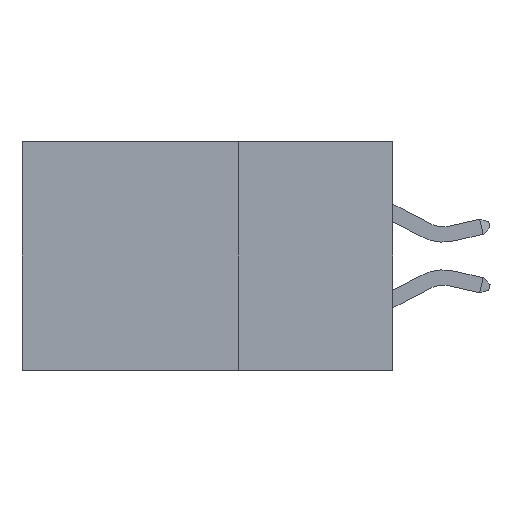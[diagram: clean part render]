
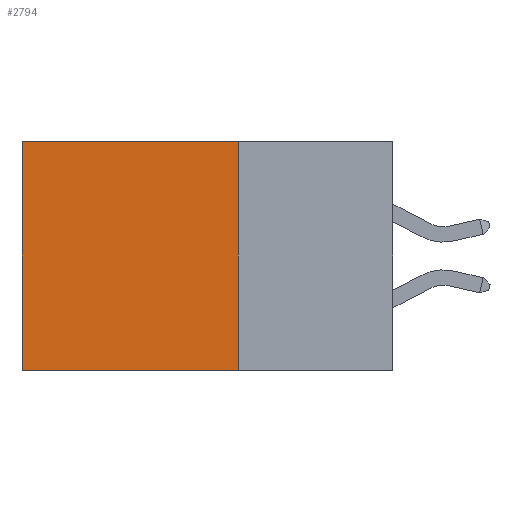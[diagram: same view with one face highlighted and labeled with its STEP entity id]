
A CAD part, left-side view. The second image highlights one B-rep face of the part: STEP entity #2794.
In plain terms, the highlighted planar face has unit normal (-1, 0, 0).
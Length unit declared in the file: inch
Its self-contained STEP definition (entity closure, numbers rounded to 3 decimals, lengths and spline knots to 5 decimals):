
#591 = CARTESIAN_POINT ( 'NONE',  ( 0.2875, 0.6, 0. ) ) ;
#1231 = ORIENTED_EDGE ( 'NONE', *, *, #15293, .T. ) ;
#2356 = DIRECTION ( 'NONE',  ( 0., 0., -1. ) ) ;
#2794 = ADVANCED_FACE ( 'NONE', ( #4543 ), #17885, .F. ) ;
#3355 = VECTOR ( 'NONE', #13983, 39.37008 ) ;
#4543 = FACE_OUTER_BOUND ( 'NONE', #29077, .T. ) ;
#4816 = CARTESIAN_POINT ( 'NONE',  ( 0.2875, 0.25, 0. ) ) ;
#7185 = CARTESIAN_POINT ( 'NONE',  ( 0.2875, 0.25, -0.37 ) ) ;
#7230 = VERTEX_POINT ( 'NONE', #27757 ) ;
#7694 = CARTESIAN_POINT ( 'NONE',  ( 0.2875, 0.6, -0.37 ) ) ;
#7785 = EDGE_CURVE ( 'NONE', #26499, #25138, #21402, .T. ) ;
#8423 = ORIENTED_EDGE ( 'NONE', *, *, #19482, .F. ) ;
#8565 = VECTOR ( 'NONE', #23103, 39.37008 ) ;
#8801 = CARTESIAN_POINT ( 'NONE',  ( 0.2875, 0.25, 0. ) ) ;
#11201 = AXIS2_PLACEMENT_3D ( 'NONE', #8801, #24836, #2356 ) ;
#11332 = DIRECTION ( 'NONE',  ( 0., 0., -1. ) ) ;
#11420 = DIRECTION ( 'NONE',  ( 0., 0., -1. ) ) ;
#12532 = CARTESIAN_POINT ( 'NONE',  ( 0.2875, 0.25, -0.37 ) ) ;
#13983 = DIRECTION ( 'NONE',  ( 0., 1., 0. ) ) ;
#15293 = EDGE_CURVE ( 'NONE', #24431, #25138, #18351, .T. ) ;
#17885 = PLANE ( 'NONE',  #11201 ) ;
#18351 = LINE ( 'NONE', #27538, #22926 ) ;
#19482 = EDGE_CURVE ( 'NONE', #7230, #26499, #23538, .T. ) ;
#21134 = CARTESIAN_POINT ( 'NONE',  ( 0.2875, 0.25, 0. ) ) ;
#21402 = LINE ( 'NONE', #7185, #3355 ) ;
#22926 = VECTOR ( 'NONE', #11420, 39.37008 ) ;
#23103 = DIRECTION ( 'NONE',  ( 0., 1., 0. ) ) ;
#23538 = LINE ( 'NONE', #4816, #24603 ) ;
#23799 = LINE ( 'NONE', #21134, #8565 ) ;
#24389 = EDGE_CURVE ( 'NONE', #7230, #24431, #23799, .T. ) ;
#24431 = VERTEX_POINT ( 'NONE', #591 ) ;
#24603 = VECTOR ( 'NONE', #11332, 39.37008 ) ;
#24836 = DIRECTION ( 'NONE',  ( 1., 0., 0. ) ) ;
#25138 = VERTEX_POINT ( 'NONE', #7694 ) ;
#25265 = ORIENTED_EDGE ( 'NONE', *, *, #7785, .F. ) ;
#26499 = VERTEX_POINT ( 'NONE', #12532 ) ;
#27538 = CARTESIAN_POINT ( 'NONE',  ( 0.2875, 0.6, 0. ) ) ;
#27757 = CARTESIAN_POINT ( 'NONE',  ( 0.2875, 0.25, 0. ) ) ;
#29040 = ORIENTED_EDGE ( 'NONE', *, *, #24389, .T. ) ;
#29077 = EDGE_LOOP ( 'NONE', ( #1231, #25265, #8423, #29040 ) ) ;
